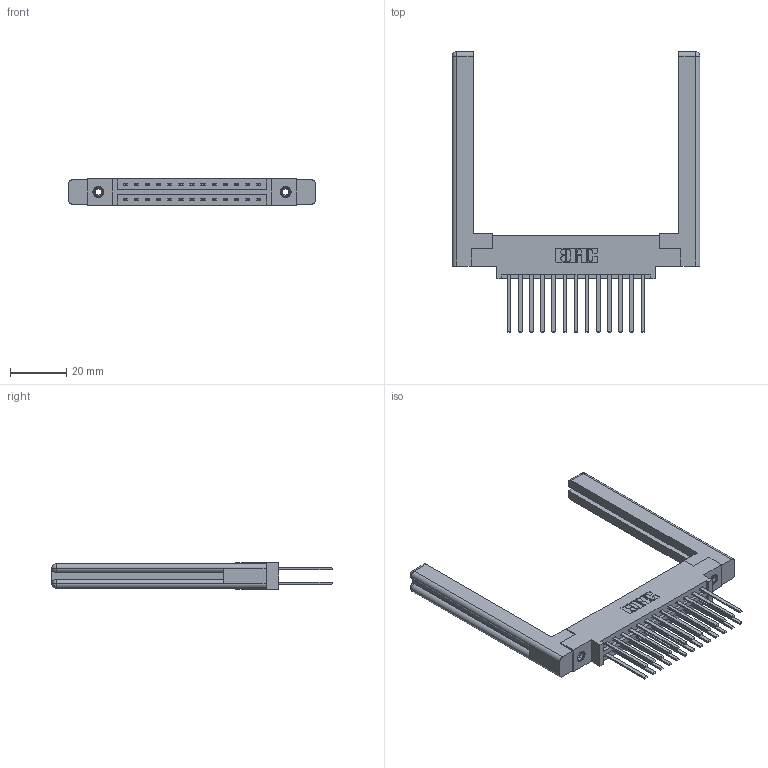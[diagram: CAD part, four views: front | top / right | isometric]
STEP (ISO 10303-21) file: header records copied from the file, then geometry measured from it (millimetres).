
FILE_DESCRIPTION (( 'STEP AP203' ), '1' );
FILE_NAME ('387-026-544-858.STEP', '2019-10-16T20:29:24', ( '' ), ( '' ), 'SwSTEP 2.0', 'SolidWorks 2016', '' );
FILE_SCHEMA (( 'CONFIG_CONTROL_DESIGN' ));
Length unit declared in the file: inch
Products named in the file (5): 387-026-544-858; 345-292-001_345-293-144; 345-250-001_345-250-001-102; 307-220-058; 337 Part_0.170 Offset - 0.156 Dia-TI
Assembly tree (31 placements, depth 2):
  387-026-544-858
    337 Part_0.170 Offset - 0.156 Dia-TI
    345-292-001_345-293-144  x26
    345-250-001_345-250-001-102  x2
    307-220-058  x2
Bounding box: 88.14 x 99.7 x 9.4 mm (x, y, z)
Volume: 16292 mm3; surface area: 16407.2 mm2
Topology: 31 solids, 31 shells, 1508 faces, 4395 edges, 2882 vertices
Faces by surface type: plane 1042, cylinder 442, cone 12, torus 12
Entity records: 16412 total; most frequent: CARTESIAN_POINT 2797, ORIENTED_EDGE 2672, DIRECTION 2444, EDGE_CURVE 1336, LINE 1164, VECTOR 1164, VERTEX_POINT 882, AXIS2_PLACEMENT_3D 640
